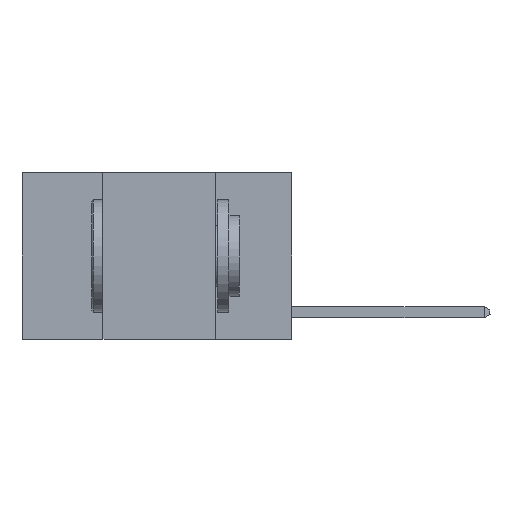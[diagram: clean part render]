
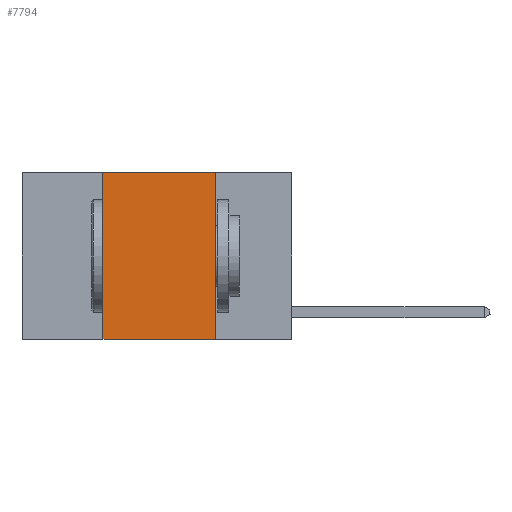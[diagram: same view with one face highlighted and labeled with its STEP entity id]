
A CAD part, left-side view. The second image highlights one B-rep face of the part: STEP entity #7794.
In plain terms, the highlighted planar face has unit normal (-1, 0, 0).
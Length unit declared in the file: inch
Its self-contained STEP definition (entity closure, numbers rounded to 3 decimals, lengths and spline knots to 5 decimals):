
#1281 = CARTESIAN_POINT ( 'NONE',  ( 0., 0.6, 0. ) ) ;
#2087 = EDGE_CURVE ( 'NONE', #12781, #4046, #9705, .T. ) ;
#3238 = DIRECTION ( 'NONE',  ( 0., -1., 0. ) ) ;
#3637 = EDGE_CURVE ( 'NONE', #8943, #7435, #15090, .T. ) ;
#4046 = VERTEX_POINT ( 'NONE', #8027 ) ;
#4081 = CARTESIAN_POINT ( 'NONE',  ( 0., 0.6, 0. ) ) ;
#4578 = LINE ( 'NONE', #1281, #7690 ) ;
#5035 = ORIENTED_EDGE ( 'NONE', *, *, #6311, .T. ) ;
#5432 = ORIENTED_EDGE ( 'NONE', *, *, #3637, .F. ) ;
#5593 = DIRECTION ( 'NONE',  ( 0., 0., 1. ) ) ;
#6181 = ORIENTED_EDGE ( 'NONE', *, *, #9728, .F. ) ;
#6311 = EDGE_CURVE ( 'NONE', #8943, #4046, #11439, .T. ) ;
#7041 = CARTESIAN_POINT ( 'NONE',  ( 0., 0.42, 0. ) ) ;
#7312 = DIRECTION ( 'NONE',  ( 0., 0., -1. ) ) ;
#7435 = VERTEX_POINT ( 'NONE', #10297 ) ;
#7690 = VECTOR ( 'NONE', #13954, 39.37008 ) ;
#7794 = ADVANCED_FACE ( 'NONE', ( #12297 ), #8547, .F. ) ;
#7953 = VECTOR ( 'NONE', #9473, 39.37008 ) ;
#8027 = CARTESIAN_POINT ( 'NONE',  ( 0., 0.17, -0.37 ) ) ;
#8197 = CARTESIAN_POINT ( 'NONE',  ( 0., 0.6, -0.37 ) ) ;
#8547 = PLANE ( 'NONE',  #14822 ) ;
#8599 = EDGE_LOOP ( 'NONE', ( #9560, #6181, #5432, #5035 ) ) ;
#8943 = VERTEX_POINT ( 'NONE', #10678 ) ;
#9473 = DIRECTION ( 'NONE',  ( 0., 0., -1. ) ) ;
#9560 = ORIENTED_EDGE ( 'NONE', *, *, #2087, .F. ) ;
#9705 = LINE ( 'NONE', #10848, #7953 ) ;
#9728 = EDGE_CURVE ( 'NONE', #7435, #12781, #4578, .T. ) ;
#10297 = CARTESIAN_POINT ( 'NONE',  ( 0., 0.42, 0. ) ) ;
#10303 = CARTESIAN_POINT ( 'NONE',  ( 0., 0.17, 0. ) ) ;
#10678 = CARTESIAN_POINT ( 'NONE',  ( 0., 0.42, -0.37 ) ) ;
#10848 = CARTESIAN_POINT ( 'NONE',  ( 0., 0.17, 0. ) ) ;
#10910 = DIRECTION ( 'NONE',  ( 1., 0., 0. ) ) ;
#11439 = LINE ( 'NONE', #8197, #13858 ) ;
#11703 = VECTOR ( 'NONE', #5593, 39.37008 ) ;
#12297 = FACE_OUTER_BOUND ( 'NONE', #8599, .T. ) ;
#12781 = VERTEX_POINT ( 'NONE', #10303 ) ;
#13858 = VECTOR ( 'NONE', #3238, 39.37008 ) ;
#13954 = DIRECTION ( 'NONE',  ( 0., -1., 0. ) ) ;
#14822 = AXIS2_PLACEMENT_3D ( 'NONE', #4081, #10910, #7312 ) ;
#15090 = LINE ( 'NONE', #7041, #11703 ) ;
